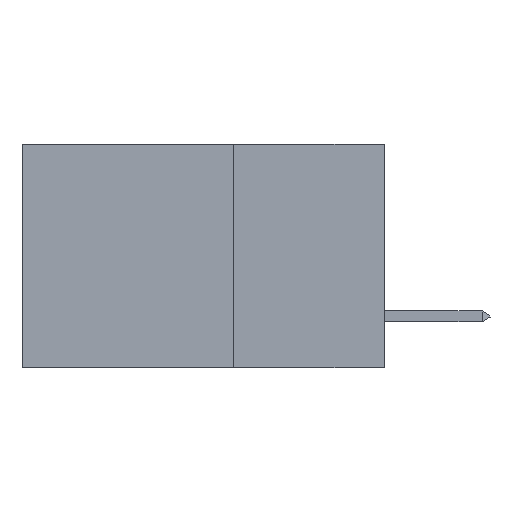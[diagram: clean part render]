
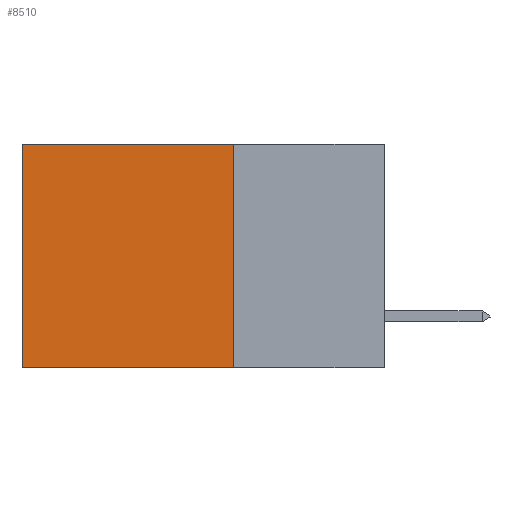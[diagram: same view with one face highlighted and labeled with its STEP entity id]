
A CAD part, left-side view. The second image highlights one B-rep face of the part: STEP entity #8510.
In plain terms, the highlighted planar face has unit normal (-1, 0, 0).
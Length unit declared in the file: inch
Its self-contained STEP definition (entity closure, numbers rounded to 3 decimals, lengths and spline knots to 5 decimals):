
#102 = CARTESIAN_POINT ( 'NONE',  ( 0.2875, 0.25, -0.37 ) ) ;
#1092 = LINE ( 'NONE', #8594, #8219 ) ;
#1537 = FACE_OUTER_BOUND ( 'NONE', #7999, .T. ) ;
#1576 = VECTOR ( 'NONE', #7625, 39.37008 ) ;
#1697 = CARTESIAN_POINT ( 'NONE',  ( 0.2875, 0.25, 0. ) ) ;
#1889 = LINE ( 'NONE', #2843, #2391 ) ;
#2030 = EDGE_CURVE ( 'NONE', #2600, #3771, #9235, .T. ) ;
#2245 = AXIS2_PLACEMENT_3D ( 'NONE', #1697, #7740, #10435 ) ;
#2391 = VECTOR ( 'NONE', #6397, 39.37008 ) ;
#2541 = PLANE ( 'NONE',  #2245 ) ;
#2600 = VERTEX_POINT ( 'NONE', #5386 ) ;
#2843 = CARTESIAN_POINT ( 'NONE',  ( 0.2875, 0.25, -0.37 ) ) ;
#3225 = CARTESIAN_POINT ( 'NONE',  ( 0.2875, 0.6, 0. ) ) ;
#3771 = VERTEX_POINT ( 'NONE', #6819 ) ;
#3920 = LINE ( 'NONE', #3225, #1576 ) ;
#4099 = CARTESIAN_POINT ( 'NONE',  ( 0.2875, 0.6, -0.37 ) ) ;
#4456 = VECTOR ( 'NONE', #9914, 39.37008 ) ;
#4674 = VERTEX_POINT ( 'NONE', #102 ) ;
#4771 = CARTESIAN_POINT ( 'NONE',  ( 0.2875, 0.25, 0. ) ) ;
#5386 = CARTESIAN_POINT ( 'NONE',  ( 0.2875, 0.25, 0. ) ) ;
#5744 = ORIENTED_EDGE ( 'NONE', *, *, #10078, .F. ) ;
#5816 = VERTEX_POINT ( 'NONE', #4099 ) ;
#5917 = DIRECTION ( 'NONE',  ( 0., 0., -1. ) ) ;
#6397 = DIRECTION ( 'NONE',  ( 0., 1., 0. ) ) ;
#6819 = CARTESIAN_POINT ( 'NONE',  ( 0.2875, 0.6, 0. ) ) ;
#7140 = EDGE_CURVE ( 'NONE', #3771, #5816, #3920, .T. ) ;
#7274 = ORIENTED_EDGE ( 'NONE', *, *, #7140, .T. ) ;
#7625 = DIRECTION ( 'NONE',  ( 0., 0., -1. ) ) ;
#7718 = ORIENTED_EDGE ( 'NONE', *, *, #9278, .F. ) ;
#7740 = DIRECTION ( 'NONE',  ( 1., 0., 0. ) ) ;
#7999 = EDGE_LOOP ( 'NONE', ( #7274, #5744, #7718, #9711 ) ) ;
#8219 = VECTOR ( 'NONE', #5917, 39.37008 ) ;
#8510 = ADVANCED_FACE ( 'NONE', ( #1537 ), #2541, .F. ) ;
#8594 = CARTESIAN_POINT ( 'NONE',  ( 0.2875, 0.25, 0. ) ) ;
#9235 = LINE ( 'NONE', #4771, #4456 ) ;
#9278 = EDGE_CURVE ( 'NONE', #2600, #4674, #1092, .T. ) ;
#9711 = ORIENTED_EDGE ( 'NONE', *, *, #2030, .T. ) ;
#9914 = DIRECTION ( 'NONE',  ( 0., 1., 0. ) ) ;
#10078 = EDGE_CURVE ( 'NONE', #4674, #5816, #1889, .T. ) ;
#10435 = DIRECTION ( 'NONE',  ( 0., 0., -1. ) ) ;
